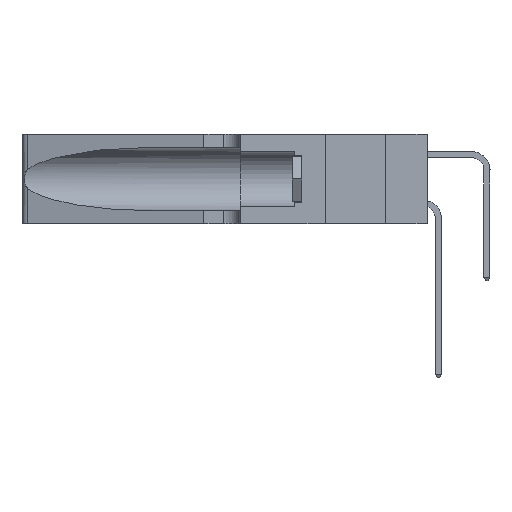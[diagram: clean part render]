
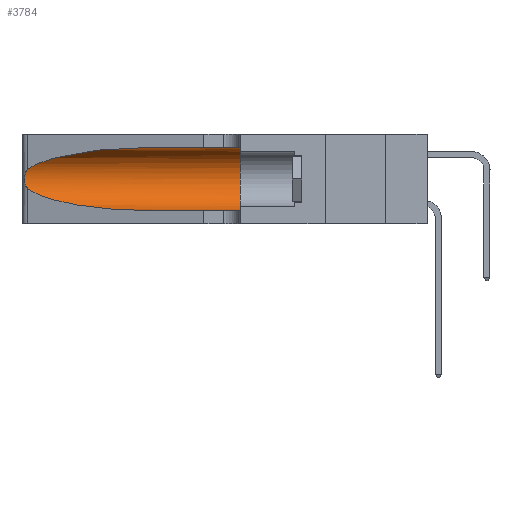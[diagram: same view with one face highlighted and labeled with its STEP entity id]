
A CAD part, left-side view. The second image highlights one B-rep face of the part: STEP entity #3784.
In plain terms, the highlighted cylindrical face has radius 3.308 mm (diameter 6.617 mm), a partial arc.
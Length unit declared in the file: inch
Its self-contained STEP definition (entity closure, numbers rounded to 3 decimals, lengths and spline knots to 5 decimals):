
#126 = CARTESIAN_POINT ( 'NONE',  ( 0.1305, 0.72297, 0.31525 ) ) ;
#270 = EDGE_CURVE ( 'NONE', #1526, #27102, #27938, .T. ) ;
#469 = DIRECTION ( 'NONE',  ( 0., -1., 0. ) ) ;
#470 = EDGE_CURVE ( 'NONE', #11815, #30801, #9861, .T. ) ;
#1526 = VERTEX_POINT ( 'NONE', #126 ) ;
#1558 = AXIS2_PLACEMENT_3D ( 'NONE', #29375, #29266, #31425 ) ;
#1934 = CARTESIAN_POINT ( 'NONE',  ( 0.1305, 1.61858, 0.185 ) ) ;
#1999 = VERTEX_POINT ( 'NONE', #16994 ) ;
#3784 = ADVANCED_FACE ( 'NONE', ( #21286 ), #15894, .F. ) ;
#4736 = CARTESIAN_POINT ( 'NONE',  ( 0.26075, 1.23896, 0.19203 ) ) ;
#5617 = VECTOR ( 'NONE', #16161, 39.37008 ) ;
#6616 = DIRECTION ( 'NONE',  ( 0., -1., 0. ) ) ;
#6852 = CARTESIAN_POINT ( 'NONE',  ( 0.25555, 1.22994, 0.2215 ) ) ;
#7129 = CARTESIAN_POINT ( 'NONE',  ( 0.18966, 0.96281, 0.31525 ) ) ;
#7594 = CARTESIAN_POINT ( 'NONE',  ( 0.1305, 1.61858, 0.31525 ) ) ;
#8670 = CARTESIAN_POINT ( 'NONE',  ( 0.1305, 1.61858, 0.05475 ) ) ;
#9301 = CARTESIAN_POINT ( 'NONE',  ( 0.25856, 1.23593, 0.16098 ) ) ;
#9475 = VERTEX_POINT ( 'NONE', #20238 ) ;
#9641 = CIRCLE ( 'NONE', #1558, 0.13025 ) ;
#9665 = CARTESIAN_POINT ( 'NONE',  ( 0.1305, 0.72297, 0.05475 ) ) ;
#9861 =( BOUNDED_CURVE ( )  B_SPLINE_CURVE ( 3, ( #29153, #14778, #14886, #9665 ),
 .UNSPECIFIED., .F., .T. ) 
 B_SPLINE_CURVE_WITH_KNOTS ( ( 4, 4 ),
 ( 3.44316, 4.71239 ),
 .UNSPECIFIED. ) 
 CURVE ( )  GEOMETRIC_REPRESENTATION_ITEM ( )  RATIONAL_B_SPLINE_CURVE ( ( 1., 0.87, 0.87, 1. ) ) 
 REPRESENTATION_ITEM ( '' )  );
#11035 = CARTESIAN_POINT ( 'NONE',  ( 0.1305, 0.72297, 0.05475 ) ) ;
#11668 = CARTESIAN_POINT ( 'NONE',  ( 0.25639, 1.23184, 0.21858 ) ) ;
#11780 = CARTESIAN_POINT ( 'NONE',  ( 0.25789, 1.23486, 0.15765 ) ) ;
#11815 = VERTEX_POINT ( 'NONE', #20306 ) ;
#12810 = B_SPLINE_CURVE_WITH_KNOTS ( 'NONE', 3,
 ( #24313, #6852, #11668, #19045, #19457, #19156, #4736, #29002, #21627, #9301, #11780, #28894, #23892, #31384 ),
 .UNSPECIFIED., .F., .F.,
 ( 4, 2, 2, 2, 2, 2, 4 ),
 ( 0., 0.00027, 0.00053, 0.00107, 0.0016, 0.00187, 0.00214 ),
 .UNSPECIFIED. ) ;
#14474 = CARTESIAN_POINT ( 'NONE',  ( 0.2373, 1.15595, 0.28018 ) ) ;
#14778 = CARTESIAN_POINT ( 'NONE',  ( 0.2373, 1.15595, 0.08982 ) ) ;
#14886 = CARTESIAN_POINT ( 'NONE',  ( 0.18966, 0.96281, 0.05475 ) ) ;
#15894 = CYLINDRICAL_SURFACE ( 'NONE', #21115, 0.13025 ) ;
#16161 = DIRECTION ( 'NONE',  ( 0., -1., 0. ) ) ;
#16938 = ORIENTED_EDGE ( 'NONE', *, *, #270, .T. ) ;
#16994 = CARTESIAN_POINT ( 'NONE',  ( 0.1305, 0.35, 0.31525 ) ) ;
#17353 = ORIENTED_EDGE ( 'NONE', *, *, #20554, .F. ) ;
#17817 = CARTESIAN_POINT ( 'NONE',  ( 0.25487, 1.22718, 0.22369 ) ) ;
#18717 = DIRECTION ( 'NONE',  ( 0., 0., -1. ) ) ;
#19045 = CARTESIAN_POINT ( 'NONE',  ( 0.25787, 1.23484, 0.2124 ) ) ;
#19124 = EDGE_CURVE ( 'NONE', #30801, #9475, #31281, .T. ) ;
#19156 = CARTESIAN_POINT ( 'NONE',  ( 0.26018, 1.23835, 0.19895 ) ) ;
#19308 = EDGE_CURVE ( 'NONE', #27102, #11815, #12810, .T. ) ;
#19457 = CARTESIAN_POINT ( 'NONE',  ( 0.25854, 1.2359, 0.20912 ) ) ;
#19621 = ORIENTED_EDGE ( 'NONE', *, *, #23478, .F. ) ;
#19625 = CARTESIAN_POINT ( 'NONE',  ( 0.1305, 0.72297, 0.31525 ) ) ;
#20233 = EDGE_LOOP ( 'NONE', ( #16938, #30237, #23373, #26938, #17353, #19621 ) ) ;
#20238 = CARTESIAN_POINT ( 'NONE',  ( 0.1305, 0.35, 0.05475 ) ) ;
#20306 = CARTESIAN_POINT ( 'NONE',  ( 0.25487, 1.22718, 0.14631 ) ) ;
#20554 = EDGE_CURVE ( 'NONE', #1999, #9475, #9641, .T. ) ;
#21115 = AXIS2_PLACEMENT_3D ( 'NONE', #1934, #6616, #18717 ) ;
#21286 = FACE_OUTER_BOUND ( 'NONE', #20233, .T. ) ;
#21321 = VECTOR ( 'NONE', #469, 39.37008 ) ;
#21627 = CARTESIAN_POINT ( 'NONE',  ( 0.26017, 1.23833, 0.17102 ) ) ;
#23373 = ORIENTED_EDGE ( 'NONE', *, *, #470, .T. ) ;
#23478 = EDGE_CURVE ( 'NONE', #1526, #1999, #31286, .T. ) ;
#23892 = CARTESIAN_POINT ( 'NONE',  ( 0.25555, 1.22993, 0.14849 ) ) ;
#24313 = CARTESIAN_POINT ( 'NONE',  ( 0.25487, 1.22718, 0.22369 ) ) ;
#24670 = CARTESIAN_POINT ( 'NONE',  ( 0.25487, 1.22718, 0.22369 ) ) ;
#26938 = ORIENTED_EDGE ( 'NONE', *, *, #19124, .T. ) ;
#27102 = VERTEX_POINT ( 'NONE', #17817 ) ;
#27938 =( BOUNDED_CURVE ( )  B_SPLINE_CURVE ( 3, ( #19625, #7129, #14474, #24670 ),
 .UNSPECIFIED., .F., .F. ) 
 B_SPLINE_CURVE_WITH_KNOTS ( ( 4, 4 ),
 ( 1.5708, 2.84003 ),
 .UNSPECIFIED. ) 
 CURVE ( )  GEOMETRIC_REPRESENTATION_ITEM ( )  RATIONAL_B_SPLINE_CURVE ( ( 1., 0.87, 0.87, 1. ) ) 
 REPRESENTATION_ITEM ( '' )  );
#28894 = CARTESIAN_POINT ( 'NONE',  ( 0.25639, 1.23186, 0.15144 ) ) ;
#29002 = CARTESIAN_POINT ( 'NONE',  ( 0.26075, 1.23896, 0.178 ) ) ;
#29153 = CARTESIAN_POINT ( 'NONE',  ( 0.25487, 1.22718, 0.14631 ) ) ;
#29266 = DIRECTION ( 'NONE',  ( 0., 1., 0. ) ) ;
#29375 = CARTESIAN_POINT ( 'NONE',  ( 0.1305, 0.35, 0.185 ) ) ;
#30237 = ORIENTED_EDGE ( 'NONE', *, *, #19308, .T. ) ;
#30801 = VERTEX_POINT ( 'NONE', #11035 ) ;
#31281 = LINE ( 'NONE', #8670, #5617 ) ;
#31286 = LINE ( 'NONE', #7594, #21321 ) ;
#31384 = CARTESIAN_POINT ( 'NONE',  ( 0.25487, 1.22718, 0.14631 ) ) ;
#31425 = DIRECTION ( 'NONE',  ( 0., 0., 1. ) ) ;
